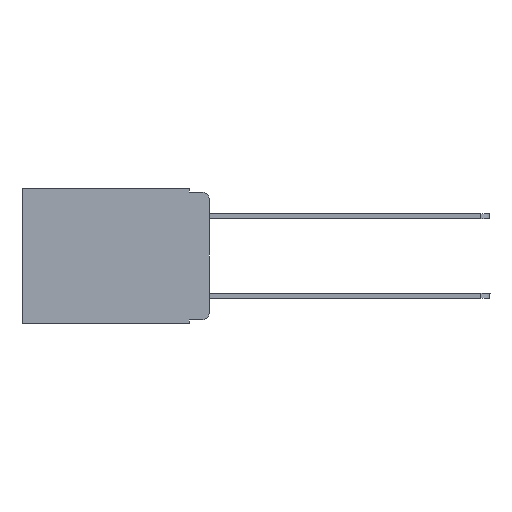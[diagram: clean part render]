
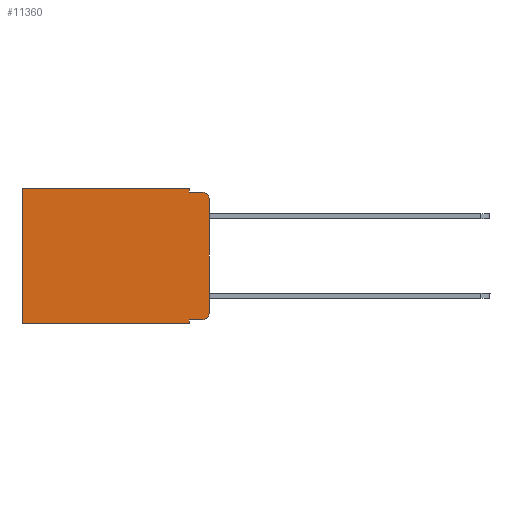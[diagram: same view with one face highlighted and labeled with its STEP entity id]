
A CAD part, left-side view. The second image highlights one B-rep face of the part: STEP entity #11360.
In plain terms, the highlighted planar face has unit normal (-1, 0, 0).
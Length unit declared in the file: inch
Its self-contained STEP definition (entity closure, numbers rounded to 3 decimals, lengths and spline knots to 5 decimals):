
#368 = EDGE_CURVE ( 'NONE', #9890, #1133, #7915, .T. ) ;
#662 = EDGE_LOOP ( 'NONE', ( #16148, #2142, #3690, #10405, #10683, #7799, #9798, #3827, #9837, #13489 ) ) ;
#794 = DIRECTION ( 'NONE',  ( 0., 0., -1. ) ) ;
#1038 = LINE ( 'NONE', #7073, #3817 ) ;
#1107 = VECTOR ( 'NONE', #15468, 39.37008 ) ;
#1133 = VERTEX_POINT ( 'NONE', #6099 ) ;
#1195 = VECTOR ( 'NONE', #3017, 39.37008 ) ;
#1426 = CARTESIAN_POINT ( 'NONE',  ( 0.298, 0.051, 0. ) ) ;
#1516 = VERTEX_POINT ( 'NONE', #3679 ) ;
#2142 = ORIENTED_EDGE ( 'NONE', *, *, #5997, .T. ) ;
#2340 = CARTESIAN_POINT ( 'NONE',  ( 0.298, 0.02, -0.313 ) ) ;
#2455 = CIRCLE ( 'NONE', #7993, 0.02 ) ;
#2462 = CARTESIAN_POINT ( 'NONE',  ( 0.298, 0., -0.313 ) ) ;
#2784 = VERTEX_POINT ( 'NONE', #9493 ) ;
#2930 = VECTOR ( 'NONE', #11374, 39.37008 ) ;
#3017 = DIRECTION ( 'NONE',  ( 0., 0., -1. ) ) ;
#3149 = EDGE_CURVE ( 'NONE', #10593, #1516, #1038, .T. ) ;
#3197 = AXIS2_PLACEMENT_3D ( 'NONE', #2340, #8701, #11342 ) ;
#3503 = AXIS2_PLACEMENT_3D ( 'NONE', #10751, #15827, #4463 ) ;
#3679 = CARTESIAN_POINT ( 'NONE',  ( 0.298, 0.051, -0.343 ) ) ;
#3690 = ORIENTED_EDGE ( 'NONE', *, *, #10753, .F. ) ;
#3817 = VECTOR ( 'NONE', #794, 39.37008 ) ;
#3826 = CARTESIAN_POINT ( 'NONE',  ( 0.298, 0., -0.343 ) ) ;
#3827 = ORIENTED_EDGE ( 'NONE', *, *, #3149, .F. ) ;
#4261 = VERTEX_POINT ( 'NONE', #2462 ) ;
#4397 = EDGE_CURVE ( 'NONE', #9890, #2784, #10394, .T. ) ;
#4404 = VECTOR ( 'NONE', #8694, 39.37008 ) ;
#4463 = DIRECTION ( 'NONE',  ( 0., 0., -1. ) ) ;
#4626 = VERTEX_POINT ( 'NONE', #10503 ) ;
#5161 = DIRECTION ( 'NONE',  ( 0., -1., 0. ) ) ;
#5524 = FACE_OUTER_BOUND ( 'NONE', #662, .T. ) ;
#5997 = EDGE_CURVE ( 'NONE', #11590, #7383, #2455, .T. ) ;
#6099 = CARTESIAN_POINT ( 'NONE',  ( 0.298, 0.473, 0. ) ) ;
#6351 = VECTOR ( 'NONE', #14593, 39.37008 ) ;
#6547 = CARTESIAN_POINT ( 'NONE',  ( 0.298, 0.051, -0.01 ) ) ;
#6617 = CIRCLE ( 'NONE', #3197, 0.02 ) ;
#7073 = CARTESIAN_POINT ( 'NONE',  ( 0.298, 0.051, 0. ) ) ;
#7383 = VERTEX_POINT ( 'NONE', #11023 ) ;
#7799 = ORIENTED_EDGE ( 'NONE', *, *, #13642, .T. ) ;
#7915 = LINE ( 'NONE', #9004, #11301 ) ;
#7964 = LINE ( 'NONE', #8052, #6351 ) ;
#7993 = AXIS2_PLACEMENT_3D ( 'NONE', #12076, #8019, #13338 ) ;
#8019 = DIRECTION ( 'NONE',  ( -1., 0., 0. ) ) ;
#8052 = CARTESIAN_POINT ( 'NONE',  ( 0.298, 0.473, 0. ) ) ;
#8535 = LINE ( 'NONE', #3826, #4404 ) ;
#8579 = LINE ( 'NONE', #13652, #2930 ) ;
#8694 = DIRECTION ( 'NONE',  ( 0., 1., 0. ) ) ;
#8701 = DIRECTION ( 'NONE',  ( -1., 0., 0. ) ) ;
#8936 = VERTEX_POINT ( 'NONE', #15112 ) ;
#8988 = EDGE_CURVE ( 'NONE', #11590, #4261, #10220, .T. ) ;
#9004 = CARTESIAN_POINT ( 'NONE',  ( 0.298, 0., 0. ) ) ;
#9493 = CARTESIAN_POINT ( 'NONE',  ( 0.298, 0.051, -0.01 ) ) ;
#9798 = ORIENTED_EDGE ( 'NONE', *, *, #10994, .F. ) ;
#9837 = ORIENTED_EDGE ( 'NONE', *, *, #11960, .T. ) ;
#9890 = VERTEX_POINT ( 'NONE', #1426 ) ;
#10081 = CARTESIAN_POINT ( 'NONE',  ( 0.298, 0., -0.03 ) ) ;
#10220 = LINE ( 'NONE', #10379, #1195 ) ;
#10379 = CARTESIAN_POINT ( 'NONE',  ( 0.298, 0., 0. ) ) ;
#10394 = LINE ( 'NONE', #10633, #1107 ) ;
#10405 = ORIENTED_EDGE ( 'NONE', *, *, #4397, .F. ) ;
#10503 = CARTESIAN_POINT ( 'NONE',  ( 0.298, 0.02, -0.333 ) ) ;
#10582 = PLANE ( 'NONE',  #3503 ) ;
#10593 = VERTEX_POINT ( 'NONE', #11281 ) ;
#10633 = CARTESIAN_POINT ( 'NONE',  ( 0.298, 0.051, 0. ) ) ;
#10683 = ORIENTED_EDGE ( 'NONE', *, *, #368, .T. ) ;
#10751 = CARTESIAN_POINT ( 'NONE',  ( 0.298, 0., 0. ) ) ;
#10753 = EDGE_CURVE ( 'NONE', #2784, #7383, #11765, .T. ) ;
#10994 = EDGE_CURVE ( 'NONE', #1516, #8936, #8535, .T. ) ;
#11023 = CARTESIAN_POINT ( 'NONE',  ( 0.298, 0.02, -0.01 ) ) ;
#11281 = CARTESIAN_POINT ( 'NONE',  ( 0.298, 0.051, -0.333 ) ) ;
#11301 = VECTOR ( 'NONE', #12908, 39.37008 ) ;
#11342 = DIRECTION ( 'NONE',  ( 0., 0., -1. ) ) ;
#11360 = ADVANCED_FACE ( 'NONE', ( #5524 ), #10582, .F. ) ;
#11374 = DIRECTION ( 'NONE',  ( 0., -1., 0. ) ) ;
#11590 = VERTEX_POINT ( 'NONE', #10081 ) ;
#11765 = LINE ( 'NONE', #6547, #16326 ) ;
#11960 = EDGE_CURVE ( 'NONE', #10593, #4626, #8579, .T. ) ;
#12076 = CARTESIAN_POINT ( 'NONE',  ( 0.298, 0.02, -0.03 ) ) ;
#12908 = DIRECTION ( 'NONE',  ( 0., 1., 0. ) ) ;
#13338 = DIRECTION ( 'NONE',  ( 0., 0., -1. ) ) ;
#13489 = ORIENTED_EDGE ( 'NONE', *, *, #13831, .T. ) ;
#13642 = EDGE_CURVE ( 'NONE', #1133, #8936, #7964, .T. ) ;
#13652 = CARTESIAN_POINT ( 'NONE',  ( 0.298, 0.051, -0.333 ) ) ;
#13831 = EDGE_CURVE ( 'NONE', #4626, #4261, #6617, .T. ) ;
#14593 = DIRECTION ( 'NONE',  ( 0., 0., -1. ) ) ;
#15112 = CARTESIAN_POINT ( 'NONE',  ( 0.298, 0.473, -0.343 ) ) ;
#15468 = DIRECTION ( 'NONE',  ( 0., 0., -1. ) ) ;
#15827 = DIRECTION ( 'NONE',  ( 1., 0., 0. ) ) ;
#16148 = ORIENTED_EDGE ( 'NONE', *, *, #8988, .F. ) ;
#16326 = VECTOR ( 'NONE', #5161, 39.37008 ) ;
